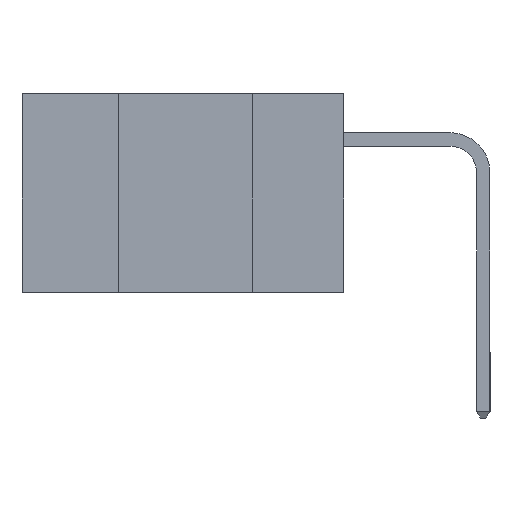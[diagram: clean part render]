
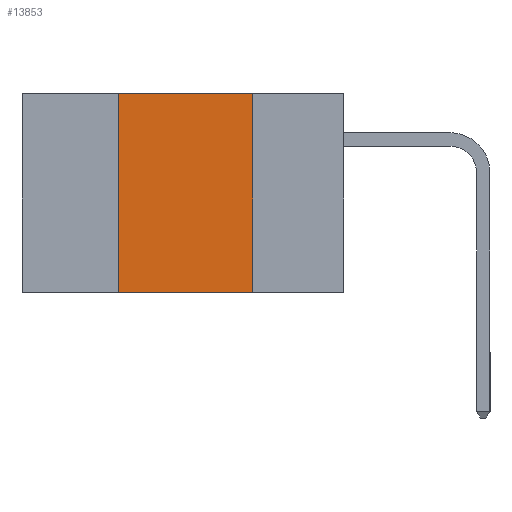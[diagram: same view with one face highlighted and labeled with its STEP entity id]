
A CAD part, left-side view. The second image highlights one B-rep face of the part: STEP entity #13853.
In plain terms, the highlighted planar face has unit normal (-1, 0, 0).
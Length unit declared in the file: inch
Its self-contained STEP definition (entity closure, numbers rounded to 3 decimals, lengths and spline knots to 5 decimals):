
#56 = VECTOR ( 'NONE', #12509, 39.37008 ) ;
#87 = VECTOR ( 'NONE', #12535, 39.37008 ) ;
#132 = VECTOR ( 'NONE', #5968, 39.37008 ) ;
#1043 = CARTESIAN_POINT ( 'NONE',  ( 0., 0.6, 0. ) ) ;
#1722 = AXIS2_PLACEMENT_3D ( 'NONE', #4287, #6790, #11718 ) ;
#1890 = PLANE ( 'NONE',  #1722 ) ;
#1909 = ORIENTED_EDGE ( 'NONE', *, *, #15490, .T. ) ;
#2260 = LINE ( 'NONE', #1043, #132 ) ;
#2661 = CARTESIAN_POINT ( 'NONE',  ( 0., 0.42, -0.37 ) ) ;
#2916 = CARTESIAN_POINT ( 'NONE',  ( 0., 0.17, -0.37 ) ) ;
#3800 = CARTESIAN_POINT ( 'NONE',  ( 0., 0.6, -0.37 ) ) ;
#4287 = CARTESIAN_POINT ( 'NONE',  ( 0., 0.6, 0. ) ) ;
#4552 = LINE ( 'NONE', #8031, #10101 ) ;
#4814 = ORIENTED_EDGE ( 'NONE', *, *, #14819, .F. ) ;
#5257 = LINE ( 'NONE', #3800, #87 ) ;
#5968 = DIRECTION ( 'NONE',  ( 0., -1., 0. ) ) ;
#6667 = EDGE_LOOP ( 'NONE', ( #4814, #11079, #8685, #1909 ) ) ;
#6685 = EDGE_CURVE ( 'NONE', #12867, #13916, #2260, .T. ) ;
#6790 = DIRECTION ( 'NONE',  ( 1., 0., 0. ) ) ;
#7800 = CARTESIAN_POINT ( 'NONE',  ( 0., 0.42, -0.37 ) ) ;
#7847 = CARTESIAN_POINT ( 'NONE',  ( 0., 0.17, 0. ) ) ;
#8031 = CARTESIAN_POINT ( 'NONE',  ( 0., 0.17, -0.37 ) ) ;
#8109 = DIRECTION ( 'NONE',  ( 0., 0., -1. ) ) ;
#8112 = EDGE_CURVE ( 'NONE', #8315, #12867, #11201, .T. ) ;
#8315 = VERTEX_POINT ( 'NONE', #7800 ) ;
#8685 = ORIENTED_EDGE ( 'NONE', *, *, #8112, .F. ) ;
#8972 = FACE_OUTER_BOUND ( 'NONE', #6667, .T. ) ;
#10101 = VECTOR ( 'NONE', #8109, 39.37008 ) ;
#11079 = ORIENTED_EDGE ( 'NONE', *, *, #6685, .F. ) ;
#11201 = LINE ( 'NONE', #2661, #56 ) ;
#11718 = DIRECTION ( 'NONE',  ( 0., 0., -1. ) ) ;
#12509 = DIRECTION ( 'NONE',  ( 0., 0., 1. ) ) ;
#12535 = DIRECTION ( 'NONE',  ( 0., -1., 0. ) ) ;
#12867 = VERTEX_POINT ( 'NONE', #13452 ) ;
#13452 = CARTESIAN_POINT ( 'NONE',  ( 0., 0.42, 0. ) ) ;
#13853 = ADVANCED_FACE ( 'NONE', ( #8972 ), #1890, .F. ) ;
#13916 = VERTEX_POINT ( 'NONE', #7847 ) ;
#14275 = VERTEX_POINT ( 'NONE', #2916 ) ;
#14819 = EDGE_CURVE ( 'NONE', #13916, #14275, #4552, .T. ) ;
#15490 = EDGE_CURVE ( 'NONE', #8315, #14275, #5257, .T. ) ;
